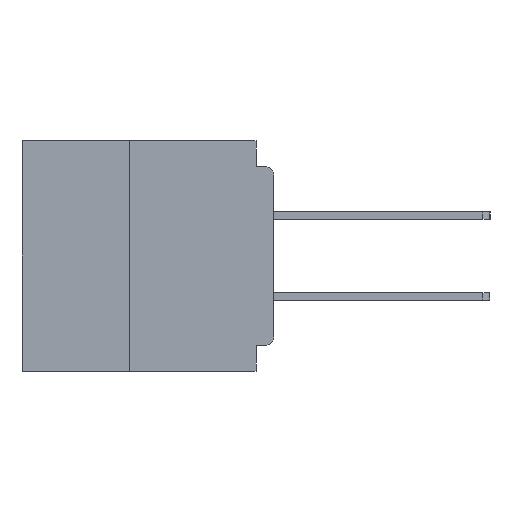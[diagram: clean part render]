
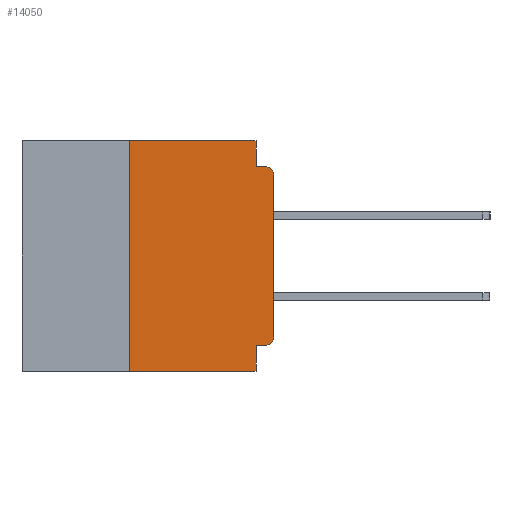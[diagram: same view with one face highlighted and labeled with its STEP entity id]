
A CAD part, left-side view. The second image highlights one B-rep face of the part: STEP entity #14050.
In plain terms, the highlighted planar face has unit normal (-1, 0, 0).
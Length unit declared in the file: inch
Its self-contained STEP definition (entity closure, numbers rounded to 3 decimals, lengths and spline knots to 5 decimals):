
#7 = CARTESIAN_POINT ( 'NONE',  ( 0., 0., -0.06 ) ) ;
#46 = VECTOR ( 'NONE', #44367, 39.37008 ) ;
#341 = DIRECTION ( 'NONE',  ( 0., 1., 0. ) ) ;
#1809 = VERTEX_POINT ( 'NONE', #7 ) ;
#1912 = CARTESIAN_POINT ( 'NONE',  ( 0., 0.437, 0. ) ) ;
#3594 = VERTEX_POINT ( 'NONE', #25689 ) ;
#4660 = CARTESIAN_POINT ( 'NONE',  ( 0., 0.031, -0.355 ) ) ;
#5354 = DIRECTION ( 'NONE',  ( 0., -1., 0. ) ) ;
#5633 = VERTEX_POINT ( 'NONE', #15518 ) ;
#6539 = ORIENTED_EDGE ( 'NONE', *, *, #7667, .F. ) ;
#6560 = CARTESIAN_POINT ( 'NONE',  ( 0., 0.437, 0. ) ) ;
#7299 = CARTESIAN_POINT ( 'NONE',  ( 0., 0.25, -0.4 ) ) ;
#7667 = EDGE_CURVE ( 'NONE', #3594, #36761, #42895, .T. ) ;
#8170 = VERTEX_POINT ( 'NONE', #55036 ) ;
#9496 = DIRECTION ( 'NONE',  ( -1., 0., 0. ) ) ;
#9961 = VECTOR ( 'NONE', #47881, 39.37008 ) ;
#10287 = CARTESIAN_POINT ( 'NONE',  ( 0., 0., 0. ) ) ;
#10453 = EDGE_CURVE ( 'NONE', #1809, #20031, #11885, .T. ) ;
#11644 = CIRCLE ( 'NONE', #15307, 0.015 ) ;
#11885 = CIRCLE ( 'NONE', #28805, 0.015 ) ;
#12310 = DIRECTION ( 'NONE',  ( 0., 0., -1. ) ) ;
#13048 = CARTESIAN_POINT ( 'NONE',  ( 0., 0., -0.355 ) ) ;
#13683 = EDGE_CURVE ( 'NONE', #8170, #38589, #30947, .T. ) ;
#14050 = ADVANCED_FACE ( 'NONE', ( #47924 ), #19064, .F. ) ;
#15307 = AXIS2_PLACEMENT_3D ( 'NONE', #35045, #9496, #39314 ) ;
#15356 = EDGE_LOOP ( 'NONE', ( #25175, #53052, #43180, #35859, #37183, #51071, #18546, #35218, #6539, #40560 ) ) ;
#15477 = CARTESIAN_POINT ( 'NONE',  ( 0., 0., -0.34 ) ) ;
#15518 = CARTESIAN_POINT ( 'NONE',  ( 0., 0.031, -0.045 ) ) ;
#15692 = CARTESIAN_POINT ( 'NONE',  ( 0., 0.031, -0.4 ) ) ;
#16821 = VECTOR ( 'NONE', #5354, 39.37008 ) ;
#18163 = CARTESIAN_POINT ( 'NONE',  ( 0., 0.437, -0.4 ) ) ;
#18546 = ORIENTED_EDGE ( 'NONE', *, *, #27306, .T. ) ;
#19064 = PLANE ( 'NONE',  #21777 ) ;
#19680 = DIRECTION ( 'NONE',  ( 0., 0., -1. ) ) ;
#20031 = VERTEX_POINT ( 'NONE', #38207 ) ;
#21549 = EDGE_CURVE ( 'NONE', #26323, #1809, #32743, .T. ) ;
#21777 = AXIS2_PLACEMENT_3D ( 'NONE', #1912, #48766, #23332 ) ;
#23332 = DIRECTION ( 'NONE',  ( 0., 0., -1. ) ) ;
#24009 = DIRECTION ( 'NONE',  ( -1., 0., 0. ) ) ;
#24082 = DIRECTION ( 'NONE',  ( 0., 0., 1. ) ) ;
#24308 = VECTOR ( 'NONE', #12310, 39.37008 ) ;
#25175 = ORIENTED_EDGE ( 'NONE', *, *, #21549, .T. ) ;
#25689 = CARTESIAN_POINT ( 'NONE',  ( 0., 0.015, -0.355 ) ) ;
#25885 = EDGE_CURVE ( 'NONE', #36761, #43728, #35649, .T. ) ;
#26323 = VERTEX_POINT ( 'NONE', #15477 ) ;
#27297 = CARTESIAN_POINT ( 'NONE',  ( 0., 0.031, 0. ) ) ;
#27306 = EDGE_CURVE ( 'NONE', #52255, #43728, #45281, .T. ) ;
#28134 = LINE ( 'NONE', #30885, #16821 ) ;
#28773 = LINE ( 'NONE', #40920, #38761 ) ;
#28805 = AXIS2_PLACEMENT_3D ( 'NONE', #49435, #24009, #53682 ) ;
#29944 = CARTESIAN_POINT ( 'NONE',  ( 0., 0.25, -0.4 ) ) ;
#30885 = CARTESIAN_POINT ( 'NONE',  ( 0., 0., -0.045 ) ) ;
#30947 = LINE ( 'NONE', #6560, #50811 ) ;
#31570 = VECTOR ( 'NONE', #341, 39.37008 ) ;
#31827 = EDGE_CURVE ( 'NONE', #5633, #20031, #28134, .T. ) ;
#32058 = EDGE_CURVE ( 'NONE', #38589, #5633, #28773, .T. ) ;
#32743 = LINE ( 'NONE', #10287, #46 ) ;
#33562 = CARTESIAN_POINT ( 'NONE',  ( 0., 0.031, -0.4 ) ) ;
#35045 = CARTESIAN_POINT ( 'NONE',  ( 0., 0.015, -0.34 ) ) ;
#35218 = ORIENTED_EDGE ( 'NONE', *, *, #25885, .F. ) ;
#35649 = LINE ( 'NONE', #33562, #24308 ) ;
#35859 = ORIENTED_EDGE ( 'NONE', *, *, #32058, .F. ) ;
#36761 = VERTEX_POINT ( 'NONE', #4660 ) ;
#37183 = ORIENTED_EDGE ( 'NONE', *, *, #13683, .F. ) ;
#37693 = LINE ( 'NONE', #7299, #47626 ) ;
#38207 = CARTESIAN_POINT ( 'NONE',  ( 0., 0.015, -0.045 ) ) ;
#38589 = VERTEX_POINT ( 'NONE', #27297 ) ;
#38761 = VECTOR ( 'NONE', #19680, 39.37008 ) ;
#39289 = EDGE_CURVE ( 'NONE', #52255, #8170, #37693, .T. ) ;
#39314 = DIRECTION ( 'NONE',  ( 0., 0., -1. ) ) ;
#39605 = EDGE_CURVE ( 'NONE', #3594, #26323, #11644, .T. ) ;
#40560 = ORIENTED_EDGE ( 'NONE', *, *, #39605, .T. ) ;
#40920 = CARTESIAN_POINT ( 'NONE',  ( 0., 0.031, 0. ) ) ;
#42895 = LINE ( 'NONE', #13048, #31570 ) ;
#43180 = ORIENTED_EDGE ( 'NONE', *, *, #31827, .F. ) ;
#43728 = VERTEX_POINT ( 'NONE', #15692 ) ;
#44367 = DIRECTION ( 'NONE',  ( 0., 0., 1. ) ) ;
#45281 = LINE ( 'NONE', #18163, #9961 ) ;
#47626 = VECTOR ( 'NONE', #24082, 39.37008 ) ;
#47881 = DIRECTION ( 'NONE',  ( 0., -1., 0. ) ) ;
#47924 = FACE_OUTER_BOUND ( 'NONE', #15356, .T. ) ;
#48766 = DIRECTION ( 'NONE',  ( 1., 0., 0. ) ) ;
#49143 = DIRECTION ( 'NONE',  ( 0., -1., 0. ) ) ;
#49435 = CARTESIAN_POINT ( 'NONE',  ( 0., 0.015, -0.06 ) ) ;
#50811 = VECTOR ( 'NONE', #49143, 39.37008 ) ;
#51071 = ORIENTED_EDGE ( 'NONE', *, *, #39289, .F. ) ;
#52255 = VERTEX_POINT ( 'NONE', #29944 ) ;
#53052 = ORIENTED_EDGE ( 'NONE', *, *, #10453, .T. ) ;
#53682 = DIRECTION ( 'NONE',  ( 0., 0., -1. ) ) ;
#55036 = CARTESIAN_POINT ( 'NONE',  ( 0., 0.25, 0. ) ) ;
